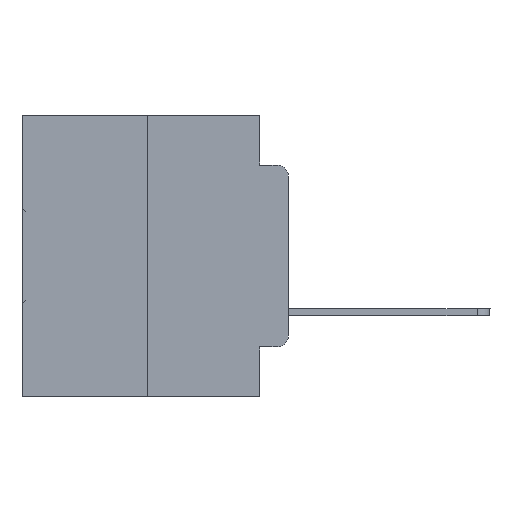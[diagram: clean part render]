
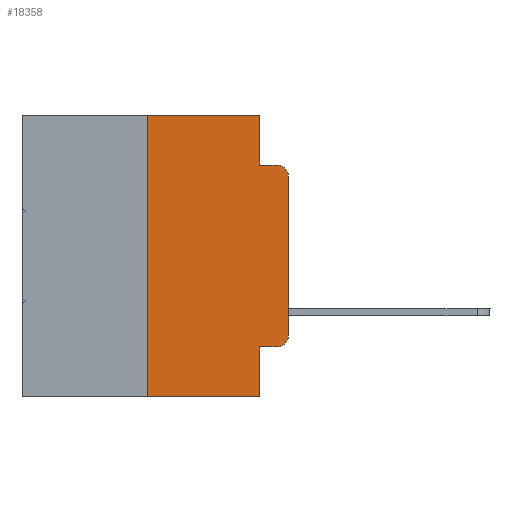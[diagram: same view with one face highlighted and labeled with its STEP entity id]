
A CAD part, left-side view. The second image highlights one B-rep face of the part: STEP entity #18358.
In plain terms, the highlighted planar face has unit normal (-1, 0, 0).
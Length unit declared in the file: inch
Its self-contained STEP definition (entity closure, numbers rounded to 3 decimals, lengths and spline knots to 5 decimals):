
#1418 = LINE ( 'NONE', #6548, #4198 ) ;
#2158 = ORIENTED_EDGE ( 'NONE', *, *, #8482, .T. ) ;
#2337 = EDGE_CURVE ( 'NONE', #19311, #19372, #29429, .T. ) ;
#2672 = EDGE_LOOP ( 'NONE', ( #2158, #23621, #24194, #14901, #30580, #15567, #30141, #7864, #16956, #22023 ) ) ;
#2757 = CARTESIAN_POINT ( 'NONE',  ( 0., 0.051, -0.5 ) ) ;
#3681 = VERTEX_POINT ( 'NONE', #26075 ) ;
#3850 = DIRECTION ( 'NONE',  ( 0., -1., 0. ) ) ;
#4198 = VECTOR ( 'NONE', #31370, 39.37008 ) ;
#4750 = VECTOR ( 'NONE', #21296, 39.37008 ) ;
#4807 = VERTEX_POINT ( 'NONE', #12369 ) ;
#5292 = CIRCLE ( 'NONE', #14268, 0.02 ) ;
#5686 = LINE ( 'NONE', #26054, #7415 ) ;
#6078 = VERTEX_POINT ( 'NONE', #22187 ) ;
#6525 = LINE ( 'NONE', #14144, #30961 ) ;
#6548 = CARTESIAN_POINT ( 'NONE',  ( 0., 0.051, -0.0885 ) ) ;
#7415 = VECTOR ( 'NONE', #3850, 39.37008 ) ;
#7864 = ORIENTED_EDGE ( 'NONE', *, *, #2337, .F. ) ;
#8228 = VERTEX_POINT ( 'NONE', #27589 ) ;
#8482 = EDGE_CURVE ( 'NONE', #8228, #9390, #6525, .T. ) ;
#9031 = CARTESIAN_POINT ( 'NONE',  ( 0., 0.473, 0. ) ) ;
#9390 = VERTEX_POINT ( 'NONE', #10930 ) ;
#9551 = LINE ( 'NONE', #9874, #23710 ) ;
#9874 = CARTESIAN_POINT ( 'NONE',  ( 0., 0.473, 0. ) ) ;
#10095 = VERTEX_POINT ( 'NONE', #12956 ) ;
#10930 = CARTESIAN_POINT ( 'NONE',  ( 0., 0., -0.1085 ) ) ;
#11510 = FACE_OUTER_BOUND ( 'NONE', #2672, .T. ) ;
#12165 = EDGE_CURVE ( 'NONE', #6078, #4807, #9551, .T. ) ;
#12196 = DIRECTION ( 'NONE',  ( 0., 0., -1. ) ) ;
#12252 = EDGE_CURVE ( 'NONE', #4807, #21085, #28085, .T. ) ;
#12369 = CARTESIAN_POINT ( 'NONE',  ( 0., 0.051, 0. ) ) ;
#12502 = CIRCLE ( 'NONE', #18882, 0.02 ) ;
#12956 = CARTESIAN_POINT ( 'NONE',  ( 0., 0.25, -0.5 ) ) ;
#13537 = EDGE_CURVE ( 'NONE', #21085, #17965, #1418, .T. ) ;
#14144 = CARTESIAN_POINT ( 'NONE',  ( 0., 0., 0. ) ) ;
#14268 = AXIS2_PLACEMENT_3D ( 'NONE', #16161, #18654, #26263 ) ;
#14901 = ORIENTED_EDGE ( 'NONE', *, *, #12252, .F. ) ;
#15188 = EDGE_CURVE ( 'NONE', #3681, #8228, #5292, .T. ) ;
#15235 = EDGE_CURVE ( 'NONE', #10095, #19372, #21624, .T. ) ;
#15514 = DIRECTION ( 'NONE',  ( 0., 0., 1. ) ) ;
#15567 = ORIENTED_EDGE ( 'NONE', *, *, #18248, .F. ) ;
#15628 = EDGE_CURVE ( 'NONE', #19311, #3681, #5686, .T. ) ;
#15935 = AXIS2_PLACEMENT_3D ( 'NONE', #9031, #21637, #23949 ) ;
#16161 = CARTESIAN_POINT ( 'NONE',  ( 0., 0.02, -0.3915 ) ) ;
#16851 = CARTESIAN_POINT ( 'NONE',  ( 0., 0.02, -0.1085 ) ) ;
#16956 = ORIENTED_EDGE ( 'NONE', *, *, #15628, .T. ) ;
#17258 = VECTOR ( 'NONE', #29754, 39.37008 ) ;
#17965 = VERTEX_POINT ( 'NONE', #23982 ) ;
#18248 = EDGE_CURVE ( 'NONE', #10095, #6078, #26274, .T. ) ;
#18329 = DIRECTION ( 'NONE',  ( 0., 0., -1. ) ) ;
#18358 = ADVANCED_FACE ( 'NONE', ( #11510 ), #31698, .F. ) ;
#18654 = DIRECTION ( 'NONE',  ( -1., 0., 0. ) ) ;
#18882 = AXIS2_PLACEMENT_3D ( 'NONE', #16851, #19507, #12196 ) ;
#19311 = VERTEX_POINT ( 'NONE', #29594 ) ;
#19372 = VERTEX_POINT ( 'NONE', #2757 ) ;
#19507 = DIRECTION ( 'NONE',  ( -1., 0., 0. ) ) ;
#19679 = DIRECTION ( 'NONE',  ( 0., -1., 0. ) ) ;
#19684 = CARTESIAN_POINT ( 'NONE',  ( 0., 0.051, 0. ) ) ;
#20008 = VECTOR ( 'NONE', #18329, 39.37008 ) ;
#20783 = CARTESIAN_POINT ( 'NONE',  ( 0., 0.051, -0.0885 ) ) ;
#21085 = VERTEX_POINT ( 'NONE', #20783 ) ;
#21286 = DIRECTION ( 'NONE',  ( 0., 0., 1. ) ) ;
#21296 = DIRECTION ( 'NONE',  ( 0., -1., 0. ) ) ;
#21624 = LINE ( 'NONE', #28726, #4750 ) ;
#21637 = DIRECTION ( 'NONE',  ( 1., 0., 0. ) ) ;
#22023 = ORIENTED_EDGE ( 'NONE', *, *, #15188, .T. ) ;
#22187 = CARTESIAN_POINT ( 'NONE',  ( 0., 0.25, 0. ) ) ;
#23621 = ORIENTED_EDGE ( 'NONE', *, *, #25503, .T. ) ;
#23710 = VECTOR ( 'NONE', #19679, 39.37008 ) ;
#23949 = DIRECTION ( 'NONE',  ( 0., 0., -1. ) ) ;
#23982 = CARTESIAN_POINT ( 'NONE',  ( 0., 0.02, -0.0885 ) ) ;
#24194 = ORIENTED_EDGE ( 'NONE', *, *, #13537, .F. ) ;
#25503 = EDGE_CURVE ( 'NONE', #9390, #17965, #12502, .T. ) ;
#25604 = CARTESIAN_POINT ( 'NONE',  ( 0., 0.051, 0. ) ) ;
#25784 = CARTESIAN_POINT ( 'NONE',  ( 0., 0.25, 0. ) ) ;
#26054 = CARTESIAN_POINT ( 'NONE',  ( 0., 0.051, -0.4115 ) ) ;
#26075 = CARTESIAN_POINT ( 'NONE',  ( 0., 0.02, -0.4115 ) ) ;
#26263 = DIRECTION ( 'NONE',  ( 0., 0., -1. ) ) ;
#26274 = LINE ( 'NONE', #25784, #32280 ) ;
#27589 = CARTESIAN_POINT ( 'NONE',  ( 0., 0., -0.3915 ) ) ;
#28085 = LINE ( 'NONE', #25604, #20008 ) ;
#28726 = CARTESIAN_POINT ( 'NONE',  ( 0., 0.473, -0.5 ) ) ;
#29429 = LINE ( 'NONE', #19684, #17258 ) ;
#29594 = CARTESIAN_POINT ( 'NONE',  ( 0., 0.051, -0.4115 ) ) ;
#29754 = DIRECTION ( 'NONE',  ( 0., 0., -1. ) ) ;
#30141 = ORIENTED_EDGE ( 'NONE', *, *, #15235, .T. ) ;
#30580 = ORIENTED_EDGE ( 'NONE', *, *, #12165, .F. ) ;
#30961 = VECTOR ( 'NONE', #21286, 39.37008 ) ;
#31370 = DIRECTION ( 'NONE',  ( 0., -1., 0. ) ) ;
#31698 = PLANE ( 'NONE',  #15935 ) ;
#32280 = VECTOR ( 'NONE', #15514, 39.37008 ) ;
